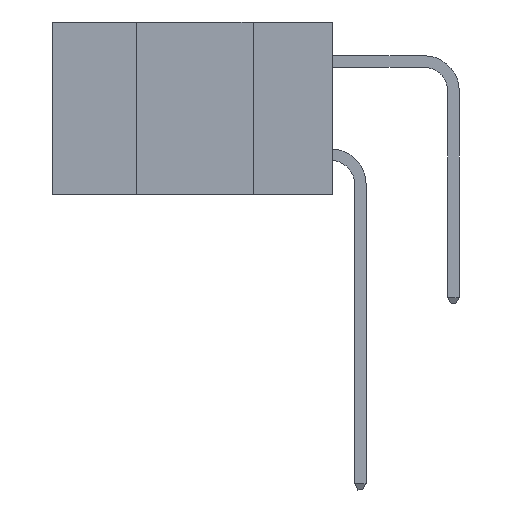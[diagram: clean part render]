
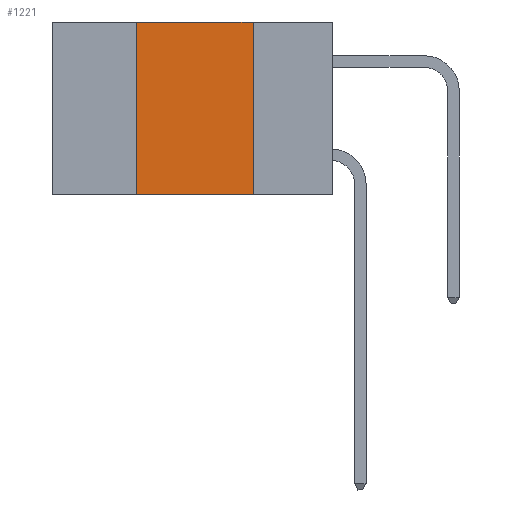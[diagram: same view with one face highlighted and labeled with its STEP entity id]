
A CAD part, left-side view. The second image highlights one B-rep face of the part: STEP entity #1221.
In plain terms, the highlighted planar face has unit normal (-1, 0, 0).
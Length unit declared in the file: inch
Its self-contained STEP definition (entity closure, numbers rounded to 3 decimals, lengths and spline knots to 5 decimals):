
#1060 = DIRECTION ( 'NONE',  ( 0., 0., 1. ) ) ;
#1137 = LINE ( 'NONE', #20162, #5739 ) ;
#1221 = ADVANCED_FACE ( 'NONE', ( #19018 ), #13523, .F. ) ;
#2807 = CARTESIAN_POINT ( 'NONE',  ( 0., 0.42, -0.37 ) ) ;
#4279 = VECTOR ( 'NONE', #12995, 39.37008 ) ;
#4315 = LINE ( 'NONE', #10933, #8842 ) ;
#4457 = VECTOR ( 'NONE', #1060, 39.37008 ) ;
#5739 = VECTOR ( 'NONE', #12530, 39.37008 ) ;
#5750 = ORIENTED_EDGE ( 'NONE', *, *, #22031, .F. ) ;
#6208 = EDGE_CURVE ( 'NONE', #15052, #6217, #4315, .T. ) ;
#6217 = VERTEX_POINT ( 'NONE', #10796 ) ;
#7601 = EDGE_LOOP ( 'NONE', ( #19765, #5750, #10832, #16534 ) ) ;
#8842 = VECTOR ( 'NONE', #10853, 39.37008 ) ;
#9218 = EDGE_CURVE ( 'NONE', #17147, #6217, #1137, .T. ) ;
#10545 = CARTESIAN_POINT ( 'NONE',  ( 0., 0.17, 0. ) ) ;
#10743 = DIRECTION ( 'NONE',  ( 1., 0., 0. ) ) ;
#10796 = CARTESIAN_POINT ( 'NONE',  ( 0., 0.17, -0.37 ) ) ;
#10832 = ORIENTED_EDGE ( 'NONE', *, *, #20754, .F. ) ;
#10853 = DIRECTION ( 'NONE',  ( 0., 0., -1. ) ) ;
#10933 = CARTESIAN_POINT ( 'NONE',  ( 0., 0.17, -0.37 ) ) ;
#11039 = CARTESIAN_POINT ( 'NONE',  ( 0., 0.6, 0. ) ) ;
#12530 = DIRECTION ( 'NONE',  ( 0., -1., 0. ) ) ;
#12995 = DIRECTION ( 'NONE',  ( 0., -1., 0. ) ) ;
#13523 = PLANE ( 'NONE',  #20965 ) ;
#13603 = CARTESIAN_POINT ( 'NONE',  ( 0., 0.6, 0. ) ) ;
#15052 = VERTEX_POINT ( 'NONE', #10545 ) ;
#16534 = ORIENTED_EDGE ( 'NONE', *, *, #9218, .T. ) ;
#17147 = VERTEX_POINT ( 'NONE', #2807 ) ;
#18363 = LINE ( 'NONE', #11039, #4279 ) ;
#19018 = FACE_OUTER_BOUND ( 'NONE', #7601, .T. ) ;
#19717 = LINE ( 'NONE', #24056, #4457 ) ;
#19765 = ORIENTED_EDGE ( 'NONE', *, *, #6208, .F. ) ;
#20162 = CARTESIAN_POINT ( 'NONE',  ( 0., 0.6, -0.37 ) ) ;
#20754 = EDGE_CURVE ( 'NONE', #17147, #22489, #19717, .T. ) ;
#20965 = AXIS2_PLACEMENT_3D ( 'NONE', #13603, #10743, #21184 ) ;
#21184 = DIRECTION ( 'NONE',  ( 0., 0., -1. ) ) ;
#22031 = EDGE_CURVE ( 'NONE', #22489, #15052, #18363, .T. ) ;
#22489 = VERTEX_POINT ( 'NONE', #23784 ) ;
#23784 = CARTESIAN_POINT ( 'NONE',  ( 0., 0.42, 0. ) ) ;
#24056 = CARTESIAN_POINT ( 'NONE',  ( 0., 0.42, -0.37 ) ) ;
